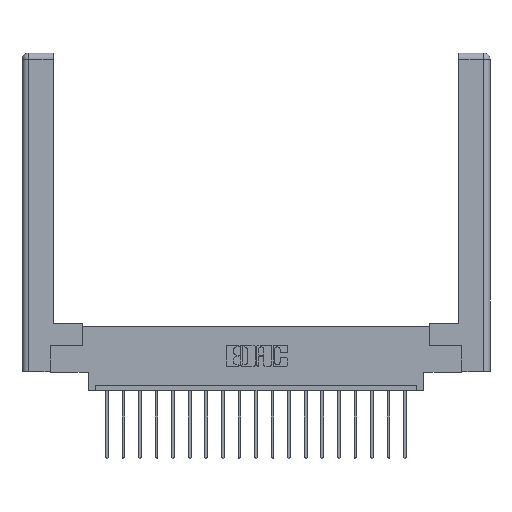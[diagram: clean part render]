
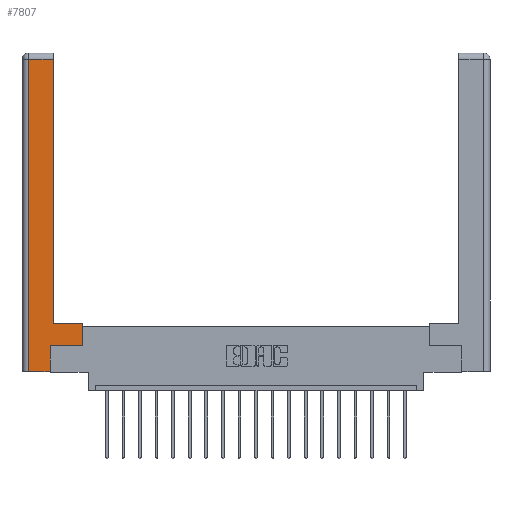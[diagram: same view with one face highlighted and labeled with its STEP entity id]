
A CAD part, top view. The second image highlights one B-rep face of the part: STEP entity #7807.
In plain terms, the highlighted planar face has unit normal (0, 0, 1).
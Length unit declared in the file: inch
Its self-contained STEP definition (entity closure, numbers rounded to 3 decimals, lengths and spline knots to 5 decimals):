
#418 = VECTOR ( 'NONE', #7469, 39.37008 ) ;
#461 = VECTOR ( 'NONE', #3120, 39.37008 ) ;
#760 = CARTESIAN_POINT ( 'NONE',  ( 0.295, 2.94, 0. ) ) ;
#880 = DIRECTION ( 'NONE',  ( -1., 0., 0. ) ) ;
#1162 = ORIENTED_EDGE ( 'NONE', *, *, #17803, .T. ) ;
#1283 = CARTESIAN_POINT ( 'NONE',  ( 0.565, 0.245, 0. ) ) ;
#1626 = AXIS2_PLACEMENT_3D ( 'NONE', #2824, #7670, #15119 ) ;
#1733 = LINE ( 'NONE', #16073, #14240 ) ;
#1962 = FACE_OUTER_BOUND ( 'NONE', #16423, .T. ) ;
#2824 = CARTESIAN_POINT ( 'NONE',  ( 0., 0., 0. ) ) ;
#2968 = ORIENTED_EDGE ( 'NONE', *, *, #13762, .T. ) ;
#3052 = VECTOR ( 'NONE', #3344, 39.37008 ) ;
#3120 = DIRECTION ( 'NONE',  ( 0., -1., 0. ) ) ;
#3344 = DIRECTION ( 'NONE',  ( -1., 0., 0. ) ) ;
#3948 = EDGE_CURVE ( 'NONE', #15216, #18289, #16286, .T. ) ;
#4957 = ORIENTED_EDGE ( 'NONE', *, *, #14285, .T. ) ;
#5158 = VERTEX_POINT ( 'NONE', #14896 ) ;
#5487 = LINE ( 'NONE', #19698, #3052 ) ;
#6222 = CARTESIAN_POINT ( 'NONE',  ( 0.265, 0., 0. ) ) ;
#7229 = EDGE_CURVE ( 'NONE', #5158, #14958, #9676, .T. ) ;
#7469 = DIRECTION ( 'NONE',  ( 0., 1., 0. ) ) ;
#7670 = DIRECTION ( 'NONE',  ( 0., 0., -1. ) ) ;
#7807 = ADVANCED_FACE ( 'NONE', ( #1962 ), #10635, .F. ) ;
#8463 = VERTEX_POINT ( 'NONE', #17606 ) ;
#8568 = LINE ( 'NONE', #14600, #12910 ) ;
#8614 = ORIENTED_EDGE ( 'NONE', *, *, #3948, .T. ) ;
#8968 = CARTESIAN_POINT ( 'NONE',  ( 0.265, 0., 0. ) ) ;
#9382 = CARTESIAN_POINT ( 'NONE',  ( 0.265, 0.245, 0. ) ) ;
#9399 = EDGE_CURVE ( 'NONE', #18289, #8463, #8568, .T. ) ;
#9676 = LINE ( 'NONE', #6222, #17116 ) ;
#9735 = VERTEX_POINT ( 'NONE', #1283 ) ;
#9789 = VECTOR ( 'NONE', #15290, 39.37008 ) ;
#10629 = CARTESIAN_POINT ( 'NONE',  ( 0.295, 3., 0. ) ) ;
#10635 = PLANE ( 'NONE',  #1626 ) ;
#10727 = CARTESIAN_POINT ( 'NONE',  ( 0.265, 0.245, 0. ) ) ;
#11023 = LINE ( 'NONE', #9382, #9789 ) ;
#11145 = CARTESIAN_POINT ( 'NONE',  ( 0.0615, 0., 0. ) ) ;
#11244 = EDGE_CURVE ( 'NONE', #9735, #17367, #1733, .T. ) ;
#11297 = ORIENTED_EDGE ( 'NONE', *, *, #9399, .T. ) ;
#11307 = LINE ( 'NONE', #11145, #461 ) ;
#11723 = DIRECTION ( 'NONE',  ( 0., 1., 0. ) ) ;
#12471 = ORIENTED_EDGE ( 'NONE', *, *, #7229, .T. ) ;
#12910 = VECTOR ( 'NONE', #880, 39.37008 ) ;
#13341 = ORIENTED_EDGE ( 'NONE', *, *, #11244, .T. ) ;
#13616 = VERTEX_POINT ( 'NONE', #10727 ) ;
#13762 = EDGE_CURVE ( 'NONE', #17367, #15216, #5487, .T. ) ;
#14051 = VECTOR ( 'NONE', #16273, 39.37008 ) ;
#14240 = VECTOR ( 'NONE', #11723, 39.37008 ) ;
#14285 = EDGE_CURVE ( 'NONE', #14958, #13616, #11023, .T. ) ;
#14600 = CARTESIAN_POINT ( 'NONE',  ( 0.0615, 2.94, 0. ) ) ;
#14896 = CARTESIAN_POINT ( 'NONE',  ( 0.0615, 0., 0. ) ) ;
#14958 = VERTEX_POINT ( 'NONE', #8968 ) ;
#15119 = DIRECTION ( 'NONE',  ( -1., 0., 0. ) ) ;
#15135 = CARTESIAN_POINT ( 'NONE',  ( 0.295, 0.45, 0. ) ) ;
#15216 = VERTEX_POINT ( 'NONE', #15135 ) ;
#15290 = DIRECTION ( 'NONE',  ( 0., 1., 0. ) ) ;
#15486 = EDGE_CURVE ( 'NONE', #13616, #9735, #15527, .T. ) ;
#15527 = LINE ( 'NONE', #17807, #14051 ) ;
#15581 = CARTESIAN_POINT ( 'NONE',  ( 0.565, 0.45, 0. ) ) ;
#16073 = CARTESIAN_POINT ( 'NONE',  ( 0.565, 0.45, 0. ) ) ;
#16273 = DIRECTION ( 'NONE',  ( 1., 0., 0. ) ) ;
#16286 = LINE ( 'NONE', #10629, #418 ) ;
#16423 = EDGE_LOOP ( 'NONE', ( #8614, #11297, #1162, #12471, #4957, #16899, #13341, #2968 ) ) ;
#16899 = ORIENTED_EDGE ( 'NONE', *, *, #15486, .T. ) ;
#17116 = VECTOR ( 'NONE', #18947, 39.37008 ) ;
#17367 = VERTEX_POINT ( 'NONE', #15581 ) ;
#17606 = CARTESIAN_POINT ( 'NONE',  ( 0.0615, 2.94, 0. ) ) ;
#17803 = EDGE_CURVE ( 'NONE', #8463, #5158, #11307, .T. ) ;
#17807 = CARTESIAN_POINT ( 'NONE',  ( 0.565, 0.245, 0. ) ) ;
#18289 = VERTEX_POINT ( 'NONE', #760 ) ;
#18947 = DIRECTION ( 'NONE',  ( 1., 0., 0. ) ) ;
#19698 = CARTESIAN_POINT ( 'NONE',  ( 0.295, 0.45, 0. ) ) ;
